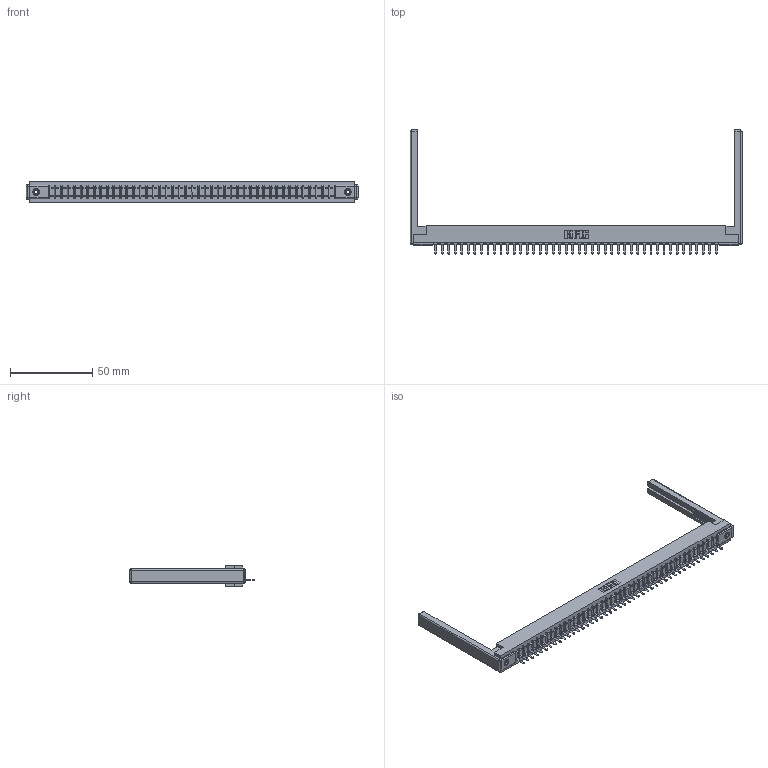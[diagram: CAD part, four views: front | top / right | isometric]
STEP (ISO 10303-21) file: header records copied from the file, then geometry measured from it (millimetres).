
FILE_DESCRIPTION (( 'STEP AP203' ), '1' );
FILE_NAME ('357-044-421-168.STEP', '2020-10-03T15:54:52', ( '' ), ( '' ), 'SwSTEP 2.0', 'SolidWorks 2020', '' );
FILE_SCHEMA (( 'CONFIG_CONTROL_DESIGN' ));
Length unit declared in the file: inch
Products named in the file (5): 307-220-068; 307-290-002_521; 345-250-001_345-250-001-102; 357-044-421-168; 307 Part_.156 Dia Mounting Holes
Assembly tree (49 placements, depth 2):
  357-044-421-168
    307 Part_.156 Dia Mounting Holes
    307-290-002_521  x44
    307-220-068  x2
    345-250-001_345-250-001-102  x2
Bounding box: 201.78 x 75.39 x 12.7 mm (x, y, z)
Volume: 25987.9 mm3; surface area: 31184 mm2
Topology: 49 solids, 49 shells, 3573 faces, 10921 edges, 7138 vertices
Faces by surface type: plane 2138, cylinder 1321, sphere 98, cone 12, torus 4
Entity records: 40951 total; most frequent: CARTESIAN_POINT 6873, ORIENTED_EDGE 6852, DIRECTION 6694, EDGE_CURVE 3426, VECTOR 2624, LINE 2624, VERTEX_POINT 2214, AXIS2_PLACEMENT_3D 2035
